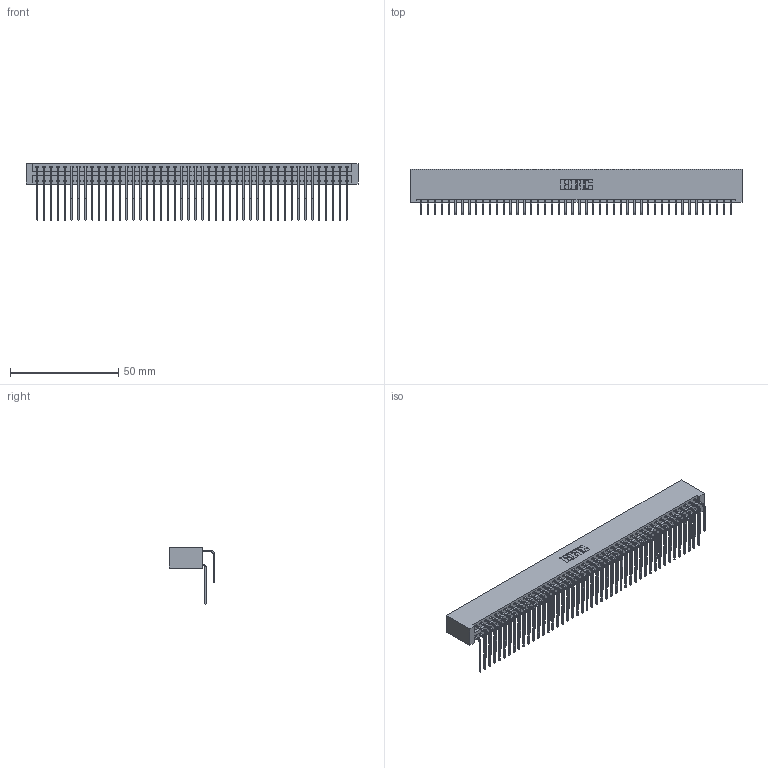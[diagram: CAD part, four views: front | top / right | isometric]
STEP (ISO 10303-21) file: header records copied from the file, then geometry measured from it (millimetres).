
FILE_DESCRIPTION (( 'STEP AP203' ), '1' );
FILE_NAME ('346-092-559-201.STEP', '2018-08-30T04:11:18', ( '' ), ( '' ), 'SwSTEP 2.0', 'SolidWorks 2016', '' );
FILE_SCHEMA (( 'CONFIG_CONTROL_DESIGN' ));
Length unit declared in the file: inch
Products named in the file (4): 345-292-001_559 Tail - 2; 346-092-559-201; 346 Part_No Mounting Lugs; 345-292-001_558 559 Tail - 1
Assembly tree (93 placements, depth 2):
  346-092-559-201
    346 Part_No Mounting Lugs
    345-292-001_558 559 Tail - 1  x46
    345-292-001_559 Tail - 2  x46
Bounding box: 153.29 x 20.89 x 26.16 mm (x, y, z)
Volume: 16082.7 mm3; surface area: 24878.8 mm2
Topology: 93 solids, 93 shells, 5082 faces, 15117 edges, 9954 vertices
Faces by surface type: plane 3476, cylinder 1606
Entity records: 30989 total; most frequent: CARTESIAN_POINT 5151, ORIENTED_EDGE 5034, DIRECTION 4557, EDGE_CURVE 2517, LINE 2169, VECTOR 2169, VERTEX_POINT 1674, AXIS2_PLACEMENT_3D 1194
